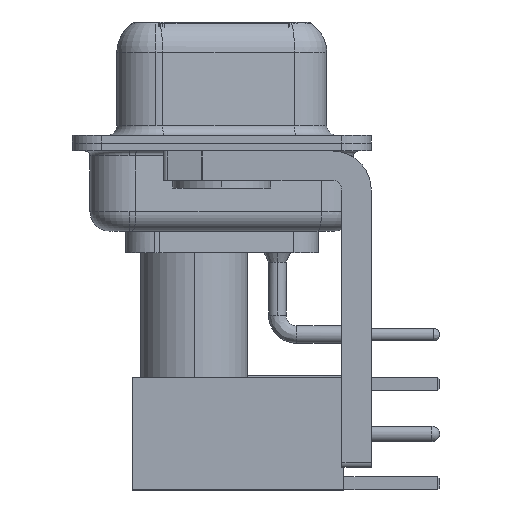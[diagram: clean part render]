
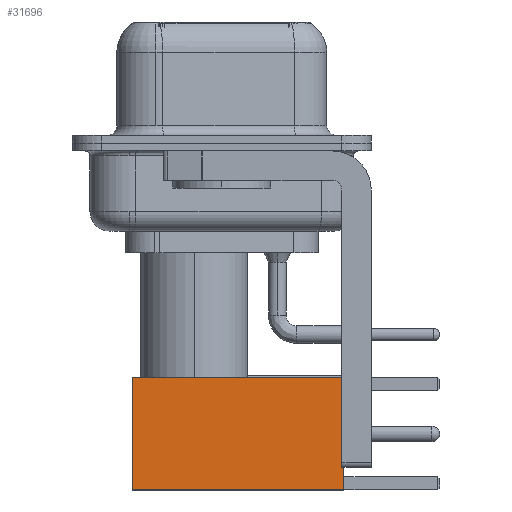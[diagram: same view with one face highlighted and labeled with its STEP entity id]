
A CAD part, left-side view. The second image highlights one B-rep face of the part: STEP entity #31696.
In plain terms, the highlighted face is planar.
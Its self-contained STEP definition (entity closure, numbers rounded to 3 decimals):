
#256 = CARTESIAN_POINT ( 'NONE',  ( 2.875, 2.875, 0. ) ) ;
#765 = LINE ( 'NONE', #14338, #24031 ) ;
#1718 = DIRECTION ( 'NONE',  ( 0., 1., 0. ) ) ;
#2303 = AXIS2_PLACEMENT_3D ( 'NONE', #4516, #1718, #35706 ) ;
#3972 = VERTEX_POINT ( 'NONE', #16664 ) ;
#4516 = CARTESIAN_POINT ( 'NONE',  ( 2.875, 2.875, 0. ) ) ;
#6312 = VERTEX_POINT ( 'NONE', #32169 ) ;
#8063 = CARTESIAN_POINT ( 'NONE',  ( 2.875, 2.875, 0. ) ) ;
#9129 = DIRECTION ( 'NONE',  ( -1., 0., 0. ) ) ;
#11095 = EDGE_CURVE ( 'NONE', #14929, #19439, #27384, .T. ) ;
#11155 = ORIENTED_EDGE ( 'NONE', *, *, #24991, .F. ) ;
#14338 = CARTESIAN_POINT ( 'NONE',  ( 0., 2.875, 10.82 ) ) ;
#14929 = VERTEX_POINT ( 'NONE', #27889 ) ;
#16664 = CARTESIAN_POINT ( 'NONE',  ( -2.875, 2.875, 10.82 ) ) ;
#16986 = CARTESIAN_POINT ( 'NONE',  ( 0., 2.875, 0. ) ) ;
#17714 = EDGE_CURVE ( 'NONE', #19439, #6312, #31613, .T. ) ;
#17878 = VECTOR ( 'NONE', #20136, 1000. ) ;
#19049 = LINE ( 'NONE', #22553, #34318 ) ;
#19439 = VERTEX_POINT ( 'NONE', #256 ) ;
#19536 = ORIENTED_EDGE ( 'NONE', *, *, #11095, .T. ) ;
#20136 = DIRECTION ( 'NONE',  ( -1., 0., 0. ) ) ;
#20350 = EDGE_LOOP ( 'NONE', ( #19536, #21560, #11155, #25642 ) ) ;
#21122 = EDGE_CURVE ( 'NONE', #14929, #3972, #765, .T. ) ;
#21422 = FACE_OUTER_BOUND ( 'NONE', #20350, .T. ) ;
#21560 = ORIENTED_EDGE ( 'NONE', *, *, #17714, .T. ) ;
#22002 = DIRECTION ( 'NONE',  ( 0., 0., -1. ) ) ;
#22553 = CARTESIAN_POINT ( 'NONE',  ( -2.875, 2.875, 0. ) ) ;
#24031 = VECTOR ( 'NONE', #9129, 1000. ) ;
#24991 = EDGE_CURVE ( 'NONE', #3972, #6312, #19049, .T. ) ;
#25642 = ORIENTED_EDGE ( 'NONE', *, *, #21122, .F. ) ;
#27384 = LINE ( 'NONE', #8063, #32998 ) ;
#27889 = CARTESIAN_POINT ( 'NONE',  ( 2.875, 2.875, 10.82 ) ) ;
#29952 = PLANE ( 'NONE',  #2303 ) ;
#30534 = DIRECTION ( 'NONE',  ( 0., 0., -1. ) ) ;
#31613 = LINE ( 'NONE', #16986, #17878 ) ;
#31696 = ADVANCED_FACE ( 'NONE', ( #21422 ), #29952, .T. ) ;
#32169 = CARTESIAN_POINT ( 'NONE',  ( -2.875, 2.875, 0. ) ) ;
#32998 = VECTOR ( 'NONE', #22002, 1000. ) ;
#34318 = VECTOR ( 'NONE', #30534, 1000. ) ;
#35706 = DIRECTION ( 'NONE',  ( 0., 0., 1. ) ) ;
